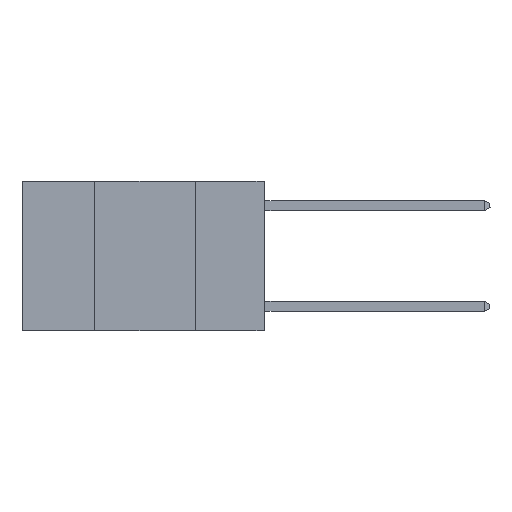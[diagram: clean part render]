
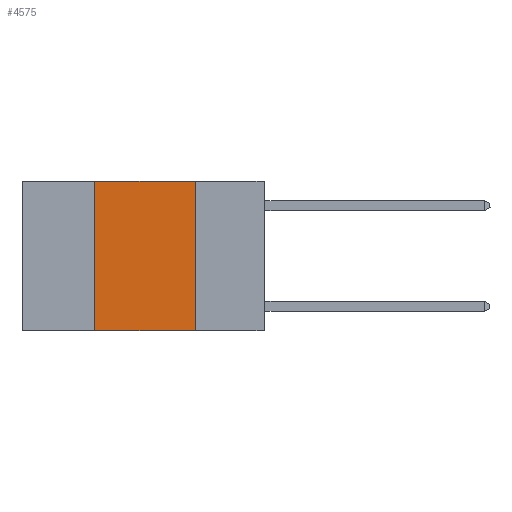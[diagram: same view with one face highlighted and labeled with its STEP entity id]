
A CAD part, left-side view. The second image highlights one B-rep face of the part: STEP entity #4575.
In plain terms, the highlighted planar face has unit normal (-1, 0, 0).
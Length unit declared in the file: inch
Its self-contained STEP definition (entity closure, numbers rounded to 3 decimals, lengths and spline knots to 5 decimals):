
#404 = VERTEX_POINT ( 'NONE', #8382 ) ;
#770 = EDGE_CURVE ( 'NONE', #12789, #404, #15270, .T. ) ;
#897 = LINE ( 'NONE', #15905, #4076 ) ;
#904 = ORIENTED_EDGE ( 'NONE', *, *, #11284, .F. ) ;
#1325 = ORIENTED_EDGE ( 'NONE', *, *, #8719, .T. ) ;
#1417 = PLANE ( 'NONE',  #7027 ) ;
#1433 = CARTESIAN_POINT ( 'NONE',  ( 0., 0.6, -0.37 ) ) ;
#1983 = VERTEX_POINT ( 'NONE', #5896 ) ;
#2054 = VECTOR ( 'NONE', #10895, 39.37008 ) ;
#2115 = EDGE_LOOP ( 'NONE', ( #3649, #4082, #904, #1325 ) ) ;
#2482 = LINE ( 'NONE', #1433, #2054 ) ;
#3649 = ORIENTED_EDGE ( 'NONE', *, *, #9457, .F. ) ;
#3657 = CARTESIAN_POINT ( 'NONE',  ( 0., 0.42, -0.37 ) ) ;
#4076 = VECTOR ( 'NONE', #6519, 39.37008 ) ;
#4082 = ORIENTED_EDGE ( 'NONE', *, *, #770, .F. ) ;
#4143 = DIRECTION ( 'NONE',  ( 1., 0., 0. ) ) ;
#4575 = ADVANCED_FACE ( 'NONE', ( #13675 ), #1417, .F. ) ;
#4884 = VERTEX_POINT ( 'NONE', #3657 ) ;
#4981 = LINE ( 'NONE', #12221, #11729 ) ;
#5896 = CARTESIAN_POINT ( 'NONE',  ( 0., 0.17, -0.37 ) ) ;
#6519 = DIRECTION ( 'NONE',  ( 0., 0., 1. ) ) ;
#7027 = AXIS2_PLACEMENT_3D ( 'NONE', #10880, #4143, #13532 ) ;
#8382 = CARTESIAN_POINT ( 'NONE',  ( 0., 0.17, 0. ) ) ;
#8719 = EDGE_CURVE ( 'NONE', #4884, #1983, #2482, .T. ) ;
#9457 = EDGE_CURVE ( 'NONE', #404, #1983, #4981, .T. ) ;
#10880 = CARTESIAN_POINT ( 'NONE',  ( 0., 0.6, 0. ) ) ;
#10895 = DIRECTION ( 'NONE',  ( 0., -1., 0. ) ) ;
#11284 = EDGE_CURVE ( 'NONE', #4884, #12789, #897, .T. ) ;
#11432 = CARTESIAN_POINT ( 'NONE',  ( 0., 0.42, 0. ) ) ;
#11726 = VECTOR ( 'NONE', #16784, 39.37008 ) ;
#11729 = VECTOR ( 'NONE', #13559, 39.37008 ) ;
#12221 = CARTESIAN_POINT ( 'NONE',  ( 0., 0.17, 0. ) ) ;
#12789 = VERTEX_POINT ( 'NONE', #11432 ) ;
#13532 = DIRECTION ( 'NONE',  ( 0., 0., -1. ) ) ;
#13559 = DIRECTION ( 'NONE',  ( 0., 0., -1. ) ) ;
#13675 = FACE_OUTER_BOUND ( 'NONE', #2115, .T. ) ;
#15270 = LINE ( 'NONE', #16917, #11726 ) ;
#15905 = CARTESIAN_POINT ( 'NONE',  ( 0., 0.42, 0. ) ) ;
#16784 = DIRECTION ( 'NONE',  ( 0., -1., 0. ) ) ;
#16917 = CARTESIAN_POINT ( 'NONE',  ( 0., 0.6, 0. ) ) ;
